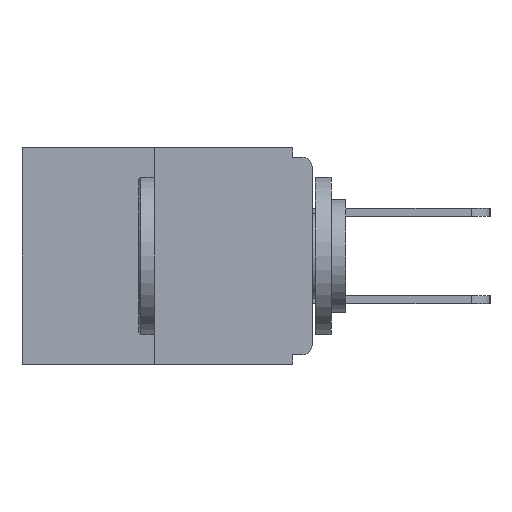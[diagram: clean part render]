
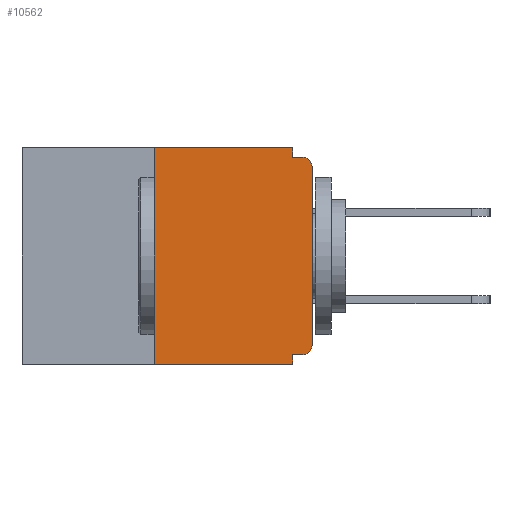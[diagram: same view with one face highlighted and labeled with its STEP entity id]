
A CAD part, left-side view. The second image highlights one B-rep face of the part: STEP entity #10562.
In plain terms, the highlighted planar face has unit normal (-1, 0, 0).
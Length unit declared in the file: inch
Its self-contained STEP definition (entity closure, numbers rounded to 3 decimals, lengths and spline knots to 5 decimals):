
#116 = CARTESIAN_POINT ( 'NONE',  ( 0., 0.015, -0.328 ) ) ;
#215 = LINE ( 'NONE', #5869, #11917 ) ;
#253 = EDGE_CURVE ( 'NONE', #580, #6267, #215, .T. ) ;
#545 = CARTESIAN_POINT ( 'NONE',  ( 0., 0.46, 0. ) ) ;
#580 = VERTEX_POINT ( 'NONE', #116 ) ;
#658 = CARTESIAN_POINT ( 'NONE',  ( 0., 0.031, -0.328 ) ) ;
#1000 = CIRCLE ( 'NONE', #11007, 0.015 ) ;
#1078 = VERTEX_POINT ( 'NONE', #18441 ) ;
#1169 = ORIENTED_EDGE ( 'NONE', *, *, #6663, .F. ) ;
#1507 = CARTESIAN_POINT ( 'NONE',  ( 0., 0., 0. ) ) ;
#1607 = ORIENTED_EDGE ( 'NONE', *, *, #12407, .T. ) ;
#1623 = ORIENTED_EDGE ( 'NONE', *, *, #16845, .F. ) ;
#1771 = VECTOR ( 'NONE', #1972, 39.37008 ) ;
#1857 = LINE ( 'NONE', #5072, #5958 ) ;
#1972 = DIRECTION ( 'NONE',  ( 0., 0., -1. ) ) ;
#2663 = DIRECTION ( 'NONE',  ( 0., 0., -1. ) ) ;
#3096 = VERTEX_POINT ( 'NONE', #22228 ) ;
#3137 = DIRECTION ( 'NONE',  ( 0., 0., 1. ) ) ;
#3390 = CARTESIAN_POINT ( 'NONE',  ( 0., 0.031, -0.015 ) ) ;
#3459 = VERTEX_POINT ( 'NONE', #21913 ) ;
#4559 = LINE ( 'NONE', #12529, #16812 ) ;
#5036 = AXIS2_PLACEMENT_3D ( 'NONE', #5950, #9404, #2663 ) ;
#5072 = CARTESIAN_POINT ( 'NONE',  ( 0., 0.25, 0. ) ) ;
#5462 = VERTEX_POINT ( 'NONE', #21153 ) ;
#5562 = VERTEX_POINT ( 'NONE', #21311 ) ;
#5621 = CARTESIAN_POINT ( 'NONE',  ( 0., 0.46, 0. ) ) ;
#5869 = CARTESIAN_POINT ( 'NONE',  ( 0., 0., -0.328 ) ) ;
#5950 = CARTESIAN_POINT ( 'NONE',  ( 0., 0.015, -0.03 ) ) ;
#5958 = VECTOR ( 'NONE', #21183, 39.37008 ) ;
#6021 = DIRECTION ( 'NONE',  ( 0., 1., 0. ) ) ;
#6079 = CARTESIAN_POINT ( 'NONE',  ( 0., 0.25, -0.343 ) ) ;
#6167 = EDGE_CURVE ( 'NONE', #7208, #1078, #1857, .T. ) ;
#6267 = VERTEX_POINT ( 'NONE', #658 ) ;
#6663 = EDGE_CURVE ( 'NONE', #19808, #5562, #4559, .T. ) ;
#7106 = CARTESIAN_POINT ( 'NONE',  ( 0., 0.46, -0.343 ) ) ;
#7208 = VERTEX_POINT ( 'NONE', #6079 ) ;
#7420 = LINE ( 'NONE', #22466, #9280 ) ;
#7463 = EDGE_CURVE ( 'NONE', #1078, #3096, #11855, .T. ) ;
#8044 = LINE ( 'NONE', #14017, #1771 ) ;
#8685 = EDGE_CURVE ( 'NONE', #10672, #5562, #15082, .T. ) ;
#9104 = ORIENTED_EDGE ( 'NONE', *, *, #14512, .F. ) ;
#9280 = VECTOR ( 'NONE', #10118, 39.37008 ) ;
#9387 = LINE ( 'NONE', #1507, #11013 ) ;
#9404 = DIRECTION ( 'NONE',  ( -1., 0., 0. ) ) ;
#9942 = LINE ( 'NONE', #7106, #12956 ) ;
#10118 = DIRECTION ( 'NONE',  ( 0., 0., -1. ) ) ;
#10427 = EDGE_CURVE ( 'NONE', #3459, #10672, #9387, .T. ) ;
#10457 = EDGE_CURVE ( 'NONE', #580, #3459, #1000, .T. ) ;
#10562 = ADVANCED_FACE ( 'NONE', ( #18729 ), #14303, .F. ) ;
#10672 = VERTEX_POINT ( 'NONE', #15336 ) ;
#10820 = DIRECTION ( 'NONE',  ( 1., 0., 0. ) ) ;
#11007 = AXIS2_PLACEMENT_3D ( 'NONE', #11796, #13849, #20548 ) ;
#11013 = VECTOR ( 'NONE', #3137, 39.37008 ) ;
#11796 = CARTESIAN_POINT ( 'NONE',  ( 0., 0.015, -0.313 ) ) ;
#11855 = LINE ( 'NONE', #545, #19207 ) ;
#11917 = VECTOR ( 'NONE', #6021, 39.37008 ) ;
#12048 = AXIS2_PLACEMENT_3D ( 'NONE', #5621, #10820, #19659 ) ;
#12407 = EDGE_CURVE ( 'NONE', #7208, #5462, #9942, .T. ) ;
#12529 = CARTESIAN_POINT ( 'NONE',  ( 0., 0., -0.015 ) ) ;
#12956 = VECTOR ( 'NONE', #15487, 39.37008 ) ;
#13842 = ORIENTED_EDGE ( 'NONE', *, *, #6167, .F. ) ;
#13849 = DIRECTION ( 'NONE',  ( -1., 0., 0. ) ) ;
#14017 = CARTESIAN_POINT ( 'NONE',  ( 0., 0.031, -0.343 ) ) ;
#14303 = PLANE ( 'NONE',  #12048 ) ;
#14512 = EDGE_CURVE ( 'NONE', #3096, #19808, #7420, .T. ) ;
#15082 = CIRCLE ( 'NONE', #5036, 0.015 ) ;
#15336 = CARTESIAN_POINT ( 'NONE',  ( 0., 0., -0.03 ) ) ;
#15487 = DIRECTION ( 'NONE',  ( 0., -1., 0. ) ) ;
#16383 = DIRECTION ( 'NONE',  ( 0., -1., 0. ) ) ;
#16615 = ORIENTED_EDGE ( 'NONE', *, *, #253, .F. ) ;
#16737 = EDGE_LOOP ( 'NONE', ( #21855, #13842, #1607, #1623, #16615, #19931, #22416, #18988, #1169, #9104 ) ) ;
#16812 = VECTOR ( 'NONE', #17588, 39.37008 ) ;
#16845 = EDGE_CURVE ( 'NONE', #6267, #5462, #8044, .T. ) ;
#17588 = DIRECTION ( 'NONE',  ( 0., -1., 0. ) ) ;
#18441 = CARTESIAN_POINT ( 'NONE',  ( 0., 0.25, 0. ) ) ;
#18729 = FACE_OUTER_BOUND ( 'NONE', #16737, .T. ) ;
#18988 = ORIENTED_EDGE ( 'NONE', *, *, #8685, .T. ) ;
#19207 = VECTOR ( 'NONE', #16383, 39.37008 ) ;
#19659 = DIRECTION ( 'NONE',  ( 0., 0., -1. ) ) ;
#19808 = VERTEX_POINT ( 'NONE', #3390 ) ;
#19931 = ORIENTED_EDGE ( 'NONE', *, *, #10457, .T. ) ;
#20548 = DIRECTION ( 'NONE',  ( 0., 0., -1. ) ) ;
#21153 = CARTESIAN_POINT ( 'NONE',  ( 0., 0.031, -0.343 ) ) ;
#21183 = DIRECTION ( 'NONE',  ( 0., 0., 1. ) ) ;
#21311 = CARTESIAN_POINT ( 'NONE',  ( 0., 0.015, -0.015 ) ) ;
#21855 = ORIENTED_EDGE ( 'NONE', *, *, #7463, .F. ) ;
#21913 = CARTESIAN_POINT ( 'NONE',  ( 0., 0., -0.313 ) ) ;
#22228 = CARTESIAN_POINT ( 'NONE',  ( 0., 0.031, 0. ) ) ;
#22416 = ORIENTED_EDGE ( 'NONE', *, *, #10427, .T. ) ;
#22466 = CARTESIAN_POINT ( 'NONE',  ( 0., 0.031, 0. ) ) ;
